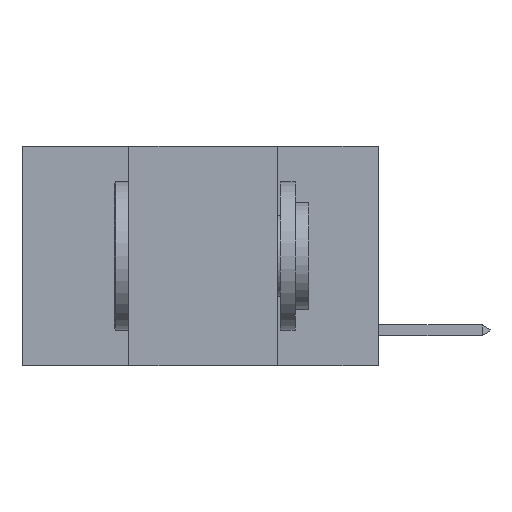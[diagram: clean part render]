
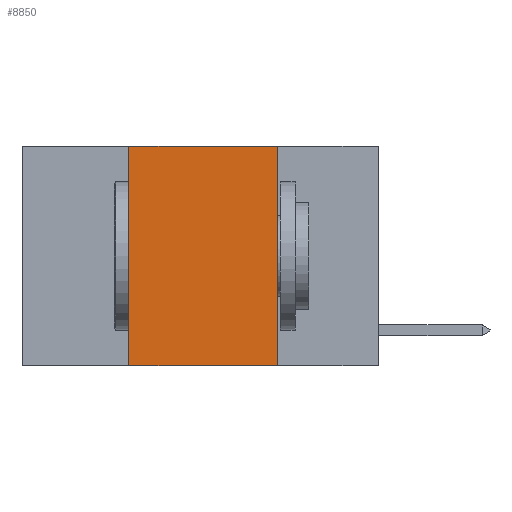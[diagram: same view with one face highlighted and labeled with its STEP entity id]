
A CAD part, left-side view. The second image highlights one B-rep face of the part: STEP entity #8850.
In plain terms, the highlighted planar face has unit normal (-1, 0, 0).
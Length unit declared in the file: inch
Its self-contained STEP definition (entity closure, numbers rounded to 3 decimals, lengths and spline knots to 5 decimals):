
#2287 = ORIENTED_EDGE ( 'NONE', *, *, #21885, .F. ) ;
#2379 = CARTESIAN_POINT ( 'NONE',  ( 0., 0.17, -0.37 ) ) ;
#2390 = VERTEX_POINT ( 'NONE', #25170 ) ;
#2743 = VECTOR ( 'NONE', #26297, 39.37008 ) ;
#3353 = EDGE_CURVE ( 'NONE', #2390, #25468, #7045, .T. ) ;
#4924 = ORIENTED_EDGE ( 'NONE', *, *, #10742, .F. ) ;
#5852 = AXIS2_PLACEMENT_3D ( 'NONE', #9066, #18235, #18383 ) ;
#6043 = LINE ( 'NONE', #22808, #25485 ) ;
#7045 = LINE ( 'NONE', #16955, #2743 ) ;
#7207 = EDGE_CURVE ( 'NONE', #25457, #15327, #10394, .T. ) ;
#7873 = CARTESIAN_POINT ( 'NONE',  ( 0., 0.17, 0. ) ) ;
#8319 = EDGE_LOOP ( 'NONE', ( #4924, #27153, #2287, #12136 ) ) ;
#8850 = ADVANCED_FACE ( 'NONE', ( #27898 ), #13480, .F. ) ;
#9066 = CARTESIAN_POINT ( 'NONE',  ( 0., 0.6, 0. ) ) ;
#10055 = VECTOR ( 'NONE', #12953, 39.37008 ) ;
#10394 = LINE ( 'NONE', #21578, #17079 ) ;
#10433 = CARTESIAN_POINT ( 'NONE',  ( 0., 0.42, -0.37 ) ) ;
#10742 = EDGE_CURVE ( 'NONE', #25468, #15327, #6043, .T. ) ;
#11755 = DIRECTION ( 'NONE',  ( 0., 0., -1. ) ) ;
#12136 = ORIENTED_EDGE ( 'NONE', *, *, #7207, .T. ) ;
#12953 = DIRECTION ( 'NONE',  ( 0., 0., 1. ) ) ;
#13480 = PLANE ( 'NONE',  #5852 ) ;
#14528 = DIRECTION ( 'NONE',  ( 0., -1., 0. ) ) ;
#15327 = VERTEX_POINT ( 'NONE', #2379 ) ;
#16955 = CARTESIAN_POINT ( 'NONE',  ( 0., 0.6, 0. ) ) ;
#17079 = VECTOR ( 'NONE', #14528, 39.37008 ) ;
#18235 = DIRECTION ( 'NONE',  ( 1., 0., 0. ) ) ;
#18383 = DIRECTION ( 'NONE',  ( 0., 0., -1. ) ) ;
#21578 = CARTESIAN_POINT ( 'NONE',  ( 0., 0.6, -0.37 ) ) ;
#21885 = EDGE_CURVE ( 'NONE', #25457, #2390, #25236, .T. ) ;
#22808 = CARTESIAN_POINT ( 'NONE',  ( 0., 0.17, 0. ) ) ;
#25170 = CARTESIAN_POINT ( 'NONE',  ( 0., 0.42, 0. ) ) ;
#25236 = LINE ( 'NONE', #27694, #10055 ) ;
#25457 = VERTEX_POINT ( 'NONE', #10433 ) ;
#25468 = VERTEX_POINT ( 'NONE', #7873 ) ;
#25485 = VECTOR ( 'NONE', #11755, 39.37008 ) ;
#26297 = DIRECTION ( 'NONE',  ( 0., -1., 0. ) ) ;
#27153 = ORIENTED_EDGE ( 'NONE', *, *, #3353, .F. ) ;
#27694 = CARTESIAN_POINT ( 'NONE',  ( 0., 0.42, 0. ) ) ;
#27898 = FACE_OUTER_BOUND ( 'NONE', #8319, .T. ) ;
